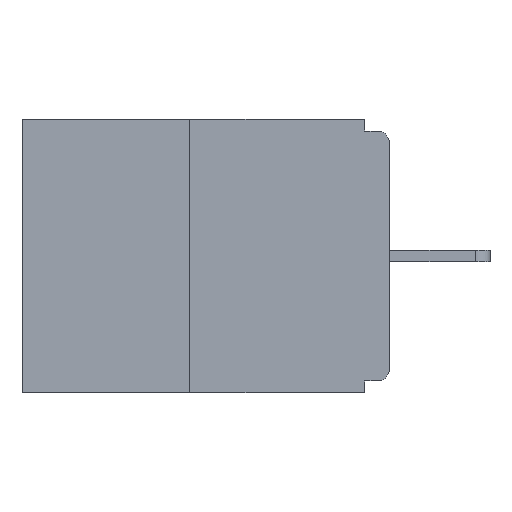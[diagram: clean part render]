
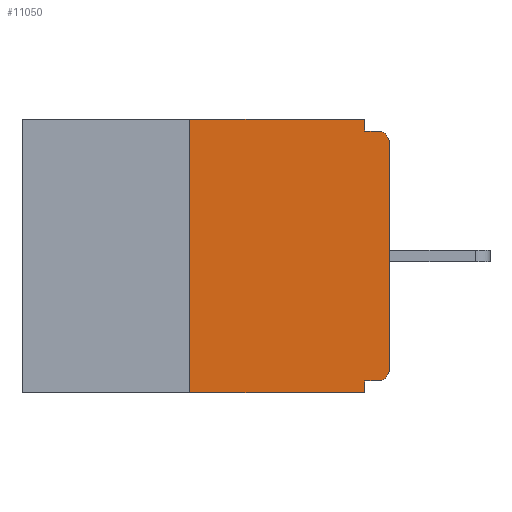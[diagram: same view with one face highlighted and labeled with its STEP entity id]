
A CAD part, left-side view. The second image highlights one B-rep face of the part: STEP entity #11050.
In plain terms, the highlighted planar face has unit normal (-1, 0, 0).
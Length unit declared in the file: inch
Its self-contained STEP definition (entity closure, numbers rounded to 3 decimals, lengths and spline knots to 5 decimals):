
#35 = VERTEX_POINT ( 'NONE', #3593 ) ;
#54 = DIRECTION ( 'NONE',  ( -1., 0., 0. ) ) ;
#56 = EDGE_CURVE ( 'NONE', #1865, #35, #5236, .T. ) ;
#190 = CARTESIAN_POINT ( 'NONE',  ( 0., 0.25, 0. ) ) ;
#284 = CARTESIAN_POINT ( 'NONE',  ( 0., 0.031, -0.343 ) ) ;
#312 = CARTESIAN_POINT ( 'NONE',  ( 0., 0.031, 0. ) ) ;
#353 = ORIENTED_EDGE ( 'NONE', *, *, #11020, .F. ) ;
#573 = DIRECTION ( 'NONE',  ( 0., 0., 1. ) ) ;
#1074 = DIRECTION ( 'NONE',  ( 0., 0., -1. ) ) ;
#1213 = EDGE_CURVE ( 'NONE', #11347, #8531, #9850, .T. ) ;
#1448 = DIRECTION ( 'NONE',  ( 0., 0., -1. ) ) ;
#1531 = LINE ( 'NONE', #190, #4288 ) ;
#1537 = DIRECTION ( 'NONE',  ( 0., -1., 0. ) ) ;
#1853 = CARTESIAN_POINT ( 'NONE',  ( 0., 0.031, 0. ) ) ;
#1865 = VERTEX_POINT ( 'NONE', #4083 ) ;
#1882 = LINE ( 'NONE', #11599, #10232 ) ;
#2051 = EDGE_CURVE ( 'NONE', #35, #11005, #11936, .T. ) ;
#2130 = VECTOR ( 'NONE', #6930, 39.37008 ) ;
#2470 = DIRECTION ( 'NONE',  ( 0., 0., 1. ) ) ;
#2521 = AXIS2_PLACEMENT_3D ( 'NONE', #7025, #54, #8185 ) ;
#2550 = CARTESIAN_POINT ( 'NONE',  ( 0., 0., -0.313 ) ) ;
#2757 = ORIENTED_EDGE ( 'NONE', *, *, #2051, .F. ) ;
#3148 = ORIENTED_EDGE ( 'NONE', *, *, #8145, .T. ) ;
#3243 = EDGE_CURVE ( 'NONE', #3587, #8111, #13876, .T. ) ;
#3294 = DIRECTION ( 'NONE',  ( 0., -1., 0. ) ) ;
#3504 = ORIENTED_EDGE ( 'NONE', *, *, #1213, .F. ) ;
#3587 = VERTEX_POINT ( 'NONE', #2550 ) ;
#3593 = CARTESIAN_POINT ( 'NONE',  ( 0., 0.031, -0.328 ) ) ;
#3823 = EDGE_CURVE ( 'NONE', #12455, #11005, #13287, .T. ) ;
#4083 = CARTESIAN_POINT ( 'NONE',  ( 0., 0.015, -0.328 ) ) ;
#4219 = CARTESIAN_POINT ( 'NONE',  ( 0., 0.25, 0. ) ) ;
#4288 = VECTOR ( 'NONE', #573, 39.37008 ) ;
#4393 = DIRECTION ( 'NONE',  ( -1., 0., 0. ) ) ;
#4598 = EDGE_CURVE ( 'NONE', #12455, #7598, #1531, .T. ) ;
#4935 = CARTESIAN_POINT ( 'NONE',  ( 0., 0., -0.328 ) ) ;
#5154 = ORIENTED_EDGE ( 'NONE', *, *, #12781, .F. ) ;
#5236 = LINE ( 'NONE', #4935, #2130 ) ;
#5277 = EDGE_LOOP ( 'NONE', ( #5154, #11018, #13675, #2757, #5848, #8871, #12545, #3148, #353, #3504 ) ) ;
#5629 = VERTEX_POINT ( 'NONE', #8759 ) ;
#5848 = ORIENTED_EDGE ( 'NONE', *, *, #56, .F. ) ;
#6139 = VECTOR ( 'NONE', #7957, 39.37008 ) ;
#6580 = CARTESIAN_POINT ( 'NONE',  ( 0., 0.46, -0.343 ) ) ;
#6871 = VECTOR ( 'NONE', #1448, 39.37008 ) ;
#6930 = DIRECTION ( 'NONE',  ( 0., 1., 0. ) ) ;
#7025 = CARTESIAN_POINT ( 'NONE',  ( 0., 0.015, -0.313 ) ) ;
#7294 = DIRECTION ( 'NONE',  ( 0., -1., 0. ) ) ;
#7338 = FACE_OUTER_BOUND ( 'NONE', #5277, .T. ) ;
#7598 = VERTEX_POINT ( 'NONE', #4219 ) ;
#7704 = VECTOR ( 'NONE', #7294, 39.37008 ) ;
#7745 = CARTESIAN_POINT ( 'NONE',  ( 0., 0., -0.03 ) ) ;
#7895 = CARTESIAN_POINT ( 'NONE',  ( 0., 0.031, -0.343 ) ) ;
#7957 = DIRECTION ( 'NONE',  ( 0., 0., -1. ) ) ;
#8036 = AXIS2_PLACEMENT_3D ( 'NONE', #14188, #8039, #1074 ) ;
#8039 = DIRECTION ( 'NONE',  ( 1., 0., 0. ) ) ;
#8111 = VERTEX_POINT ( 'NONE', #7745 ) ;
#8145 = EDGE_CURVE ( 'NONE', #8111, #5629, #12752, .T. ) ;
#8185 = DIRECTION ( 'NONE',  ( 0., 0., -1. ) ) ;
#8531 = VERTEX_POINT ( 'NONE', #12601 ) ;
#8759 = CARTESIAN_POINT ( 'NONE',  ( 0., 0.015, -0.015 ) ) ;
#8871 = ORIENTED_EDGE ( 'NONE', *, *, #9618, .T. ) ;
#9618 = EDGE_CURVE ( 'NONE', #1865, #3587, #11764, .T. ) ;
#9850 = LINE ( 'NONE', #1853, #6871 ) ;
#10232 = VECTOR ( 'NONE', #1537, 39.37008 ) ;
#10574 = CARTESIAN_POINT ( 'NONE',  ( 0., 0., -0.015 ) ) ;
#10602 = LINE ( 'NONE', #10574, #7704 ) ;
#10612 = VECTOR ( 'NONE', #3294, 39.37008 ) ;
#11005 = VERTEX_POINT ( 'NONE', #284 ) ;
#11018 = ORIENTED_EDGE ( 'NONE', *, *, #4598, .F. ) ;
#11020 = EDGE_CURVE ( 'NONE', #8531, #5629, #10602, .T. ) ;
#11040 = CARTESIAN_POINT ( 'NONE',  ( 0., 0.015, -0.03 ) ) ;
#11050 = ADVANCED_FACE ( 'NONE', ( #7338 ), #11647, .F. ) ;
#11243 = VECTOR ( 'NONE', #2470, 39.37008 ) ;
#11347 = VERTEX_POINT ( 'NONE', #312 ) ;
#11599 = CARTESIAN_POINT ( 'NONE',  ( 0., 0.46, 0. ) ) ;
#11647 = PLANE ( 'NONE',  #8036 ) ;
#11670 = AXIS2_PLACEMENT_3D ( 'NONE', #11040, #4393, #12083 ) ;
#11764 = CIRCLE ( 'NONE', #2521, 0.015 ) ;
#11936 = LINE ( 'NONE', #7895, #6139 ) ;
#12083 = DIRECTION ( 'NONE',  ( 0., 0., -1. ) ) ;
#12271 = CARTESIAN_POINT ( 'NONE',  ( 0., 0., 0. ) ) ;
#12455 = VERTEX_POINT ( 'NONE', #13217 ) ;
#12545 = ORIENTED_EDGE ( 'NONE', *, *, #3243, .T. ) ;
#12601 = CARTESIAN_POINT ( 'NONE',  ( 0., 0.031, -0.015 ) ) ;
#12752 = CIRCLE ( 'NONE', #11670, 0.015 ) ;
#12781 = EDGE_CURVE ( 'NONE', #7598, #11347, #1882, .T. ) ;
#13217 = CARTESIAN_POINT ( 'NONE',  ( 0., 0.25, -0.343 ) ) ;
#13287 = LINE ( 'NONE', #6580, #10612 ) ;
#13675 = ORIENTED_EDGE ( 'NONE', *, *, #3823, .T. ) ;
#13876 = LINE ( 'NONE', #12271, #11243 ) ;
#14188 = CARTESIAN_POINT ( 'NONE',  ( 0., 0.46, 0. ) ) ;
